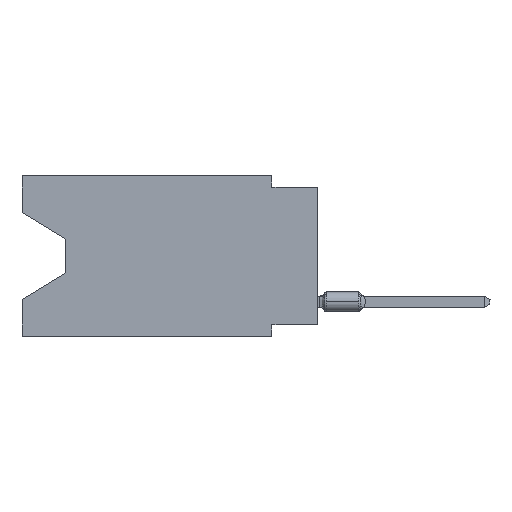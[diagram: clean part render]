
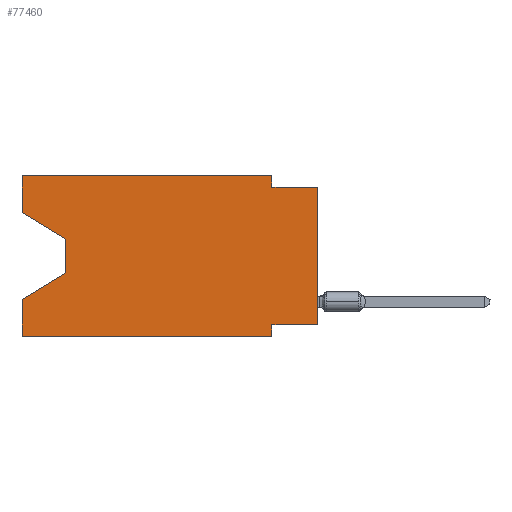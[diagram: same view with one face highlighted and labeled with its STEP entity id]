
A CAD part, left-side view. The second image highlights one B-rep face of the part: STEP entity #77460.
In plain terms, the highlighted planar face has unit normal (-1, 0, 0).
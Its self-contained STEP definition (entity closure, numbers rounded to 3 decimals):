
#2165 = CARTESIAN_POINT ( 'NONE',  ( 0., 2.54, -8.89 ) ) ;
#2241 = LINE ( 'NONE', #11287, #4255 ) ;
#2636 = DIRECTION ( 'NONE',  ( 0., 0., -1. ) ) ;
#3648 = CARTESIAN_POINT ( 'NONE',  ( 0., 2.54, 0. ) ) ;
#4255 = VECTOR ( 'NONE', #48126, 1000. ) ;
#4931 = CARTESIAN_POINT ( 'NONE',  ( 0., 13.97, -3.505 ) ) ;
#7274 = CARTESIAN_POINT ( 'NONE',  ( 0., 16.383, 0. ) ) ;
#7469 = LINE ( 'NONE', #69671, #32698 ) ;
#9604 = DIRECTION ( 'NONE',  ( 0., 0., 1. ) ) ;
#11280 = VECTOR ( 'NONE', #47079, 1000. ) ;
#11287 = CARTESIAN_POINT ( 'NONE',  ( 0., 2.54, 0. ) ) ;
#11940 = VERTEX_POINT ( 'NONE', #46020 ) ;
#12872 = VECTOR ( 'NONE', #103714, 1000. ) ;
#13403 = ORIENTED_EDGE ( 'NONE', *, *, #42825, .T. ) ;
#13975 = EDGE_CURVE ( 'NONE', #58522, #96511, #2241, .T. ) ;
#14112 = CARTESIAN_POINT ( 'NONE',  ( 0., 16.383, 0. ) ) ;
#14131 = DIRECTION ( 'NONE',  ( 0., -1., 0. ) ) ;
#14569 = VERTEX_POINT ( 'NONE', #25395 ) ;
#16311 = LINE ( 'NONE', #7274, #11280 ) ;
#16878 = LINE ( 'NONE', #62746, #81223 ) ;
#16961 = CARTESIAN_POINT ( 'NONE',  ( 0., 0., -8.255 ) ) ;
#17906 = ORIENTED_EDGE ( 'NONE', *, *, #104649, .F. ) ;
#22052 = DIRECTION ( 'NONE',  ( 0., 0., 1. ) ) ;
#24608 = VERTEX_POINT ( 'NONE', #111751 ) ;
#25395 = CARTESIAN_POINT ( 'NONE',  ( 0., 0., -0.635 ) ) ;
#27100 = VERTEX_POINT ( 'NONE', #27842 ) ;
#27842 = CARTESIAN_POINT ( 'NONE',  ( 0., 16.383, 0. ) ) ;
#28316 = CARTESIAN_POINT ( 'NONE',  ( 0., 16.383, 0. ) ) ;
#32698 = VECTOR ( 'NONE', #60630, 1000. ) ;
#33105 = VECTOR ( 'NONE', #100583, 1000. ) ;
#33724 = ORIENTED_EDGE ( 'NONE', *, *, #110005, .F. ) ;
#34025 = EDGE_CURVE ( 'NONE', #73721, #78674, #16878, .T. ) ;
#34026 = CARTESIAN_POINT ( 'NONE',  ( 0., 16.383, -6.852 ) ) ;
#36318 = ORIENTED_EDGE ( 'NONE', *, *, #78741, .F. ) ;
#38894 = EDGE_CURVE ( 'NONE', #73721, #76439, #100866, .T. ) ;
#42825 = EDGE_CURVE ( 'NONE', #103490, #54080, #48517, .T. ) ;
#44367 = ORIENTED_EDGE ( 'NONE', *, *, #13975, .F. ) ;
#46020 = CARTESIAN_POINT ( 'NONE',  ( 0., 16.383, -2.038 ) ) ;
#47079 = DIRECTION ( 'NONE',  ( 0., -1., 0. ) ) ;
#48126 = DIRECTION ( 'NONE',  ( 0., 0., -1. ) ) ;
#48168 = ORIENTED_EDGE ( 'NONE', *, *, #38894, .T. ) ;
#48517 = LINE ( 'NONE', #85278, #49978 ) ;
#49932 = CARTESIAN_POINT ( 'NONE',  ( 0., 16.383, -8.89 ) ) ;
#49978 = VECTOR ( 'NONE', #2636, 1000. ) ;
#53621 = EDGE_CURVE ( 'NONE', #67794, #24608, #54398, .T. ) ;
#54080 = VERTEX_POINT ( 'NONE', #102778 ) ;
#54398 = LINE ( 'NONE', #16961, #87891 ) ;
#55085 = VECTOR ( 'NONE', #9604, 1000. ) ;
#57739 = EDGE_CURVE ( 'NONE', #54080, #78674, #7469, .T. ) ;
#58522 = VERTEX_POINT ( 'NONE', #3648 ) ;
#59422 = VECTOR ( 'NONE', #22052, 1000. ) ;
#60630 = DIRECTION ( 'NONE',  ( 0., 0.855, -0.519 ) ) ;
#61070 = CARTESIAN_POINT ( 'NONE',  ( 0., 2.54, -0.635 ) ) ;
#61641 = EDGE_CURVE ( 'NONE', #11940, #103490, #90918, .T. ) ;
#61938 = AXIS2_PLACEMENT_3D ( 'NONE', #14112, #95612, #116088 ) ;
#62746 = CARTESIAN_POINT ( 'NONE',  ( 0., 16.383, 0. ) ) ;
#62856 = CARTESIAN_POINT ( 'NONE',  ( 0., 16.383, -8.89 ) ) ;
#64026 = EDGE_CURVE ( 'NONE', #67794, #14569, #75172, .T. ) ;
#64093 = VECTOR ( 'NONE', #14131, 1000. ) ;
#66266 = ORIENTED_EDGE ( 'NONE', *, *, #106653, .F. ) ;
#67496 = CARTESIAN_POINT ( 'NONE',  ( 0., 2.54, -8.89 ) ) ;
#67794 = VERTEX_POINT ( 'NONE', #68784 ) ;
#68784 = CARTESIAN_POINT ( 'NONE',  ( 0., 0., -8.255 ) ) ;
#69651 = CARTESIAN_POINT ( 'NONE',  ( 0., 0., -0.635 ) ) ;
#69671 = CARTESIAN_POINT ( 'NONE',  ( 0., 13.97, -5.385 ) ) ;
#73073 = DIRECTION ( 'NONE',  ( 0., 1., 0. ) ) ;
#73721 = VERTEX_POINT ( 'NONE', #49932 ) ;
#74581 = VECTOR ( 'NONE', #109915, 1000. ) ;
#74760 = LINE ( 'NONE', #28316, #55085 ) ;
#75172 = LINE ( 'NONE', #114379, #59422 ) ;
#76439 = VERTEX_POINT ( 'NONE', #2165 ) ;
#77460 = ADVANCED_FACE ( 'NONE', ( #79260 ), #96787, .F. ) ;
#77510 = LINE ( 'NONE', #69651, #64093 ) ;
#78307 = LINE ( 'NONE', #67496, #12872 ) ;
#78674 = VERTEX_POINT ( 'NONE', #34026 ) ;
#78741 = EDGE_CURVE ( 'NONE', #96511, #14569, #77510, .T. ) ;
#79260 = FACE_OUTER_BOUND ( 'NONE', #89922, .T. ) ;
#81223 = VECTOR ( 'NONE', #99561, 1000. ) ;
#83397 = ORIENTED_EDGE ( 'NONE', *, *, #34025, .F. ) ;
#85067 = ORIENTED_EDGE ( 'NONE', *, *, #57739, .T. ) ;
#85278 = CARTESIAN_POINT ( 'NONE',  ( 0., 13.97, -3.505 ) ) ;
#86049 = ORIENTED_EDGE ( 'NONE', *, *, #53621, .F. ) ;
#87891 = VECTOR ( 'NONE', #73073, 1000. ) ;
#89922 = EDGE_LOOP ( 'NONE', ( #118754, #13403, #85067, #83397, #48168, #66266, #86049, #101260, #36318, #44367, #33724, #17906 ) ) ;
#90918 = LINE ( 'NONE', #119287, #33105 ) ;
#95612 = DIRECTION ( 'NONE',  ( 1., 0., 0. ) ) ;
#96511 = VERTEX_POINT ( 'NONE', #61070 ) ;
#96787 = PLANE ( 'NONE',  #61938 ) ;
#99561 = DIRECTION ( 'NONE',  ( 0., 0., 1. ) ) ;
#100583 = DIRECTION ( 'NONE',  ( 0., -0.855, -0.519 ) ) ;
#100866 = LINE ( 'NONE', #62856, #74581 ) ;
#101260 = ORIENTED_EDGE ( 'NONE', *, *, #64026, .T. ) ;
#102778 = CARTESIAN_POINT ( 'NONE',  ( 0., 13.97, -5.385 ) ) ;
#103490 = VERTEX_POINT ( 'NONE', #4931 ) ;
#103714 = DIRECTION ( 'NONE',  ( 0., 0., -1. ) ) ;
#104649 = EDGE_CURVE ( 'NONE', #11940, #27100, #74760, .T. ) ;
#106653 = EDGE_CURVE ( 'NONE', #24608, #76439, #78307, .T. ) ;
#109915 = DIRECTION ( 'NONE',  ( 0., -1., 0. ) ) ;
#110005 = EDGE_CURVE ( 'NONE', #27100, #58522, #16311, .T. ) ;
#111751 = CARTESIAN_POINT ( 'NONE',  ( 0., 2.54, -8.255 ) ) ;
#114379 = CARTESIAN_POINT ( 'NONE',  ( 0., 0., 0. ) ) ;
#116088 = DIRECTION ( 'NONE',  ( 0., 0., -1. ) ) ;
#118754 = ORIENTED_EDGE ( 'NONE', *, *, #61641, .T. ) ;
#119287 = CARTESIAN_POINT ( 'NONE',  ( 0., 16.383, -2.038 ) ) ;
